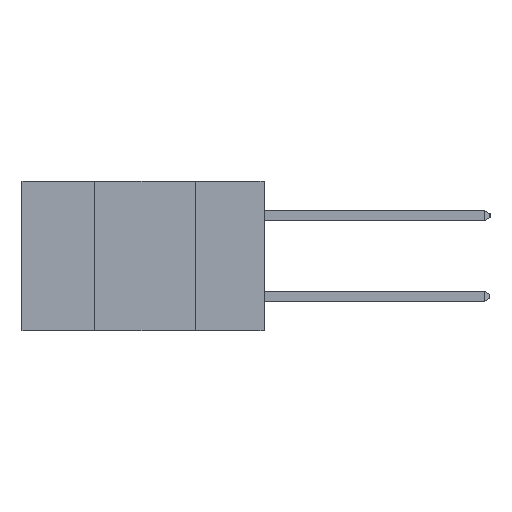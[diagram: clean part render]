
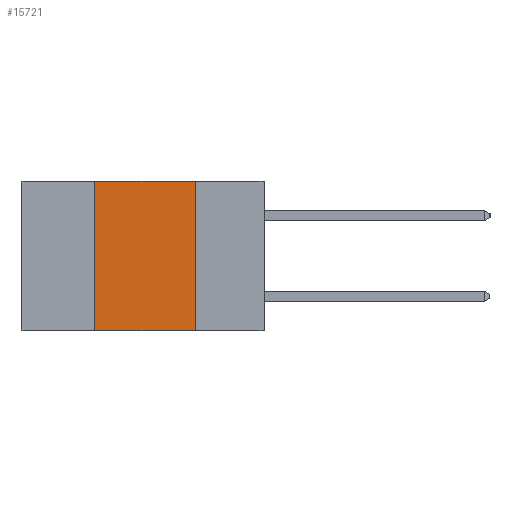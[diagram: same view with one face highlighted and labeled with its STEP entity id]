
A CAD part, left-side view. The second image highlights one B-rep face of the part: STEP entity #15721.
In plain terms, the highlighted planar face has unit normal (-1, 0, 0).
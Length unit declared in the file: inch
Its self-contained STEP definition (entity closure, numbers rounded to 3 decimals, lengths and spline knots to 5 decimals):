
#347 = VECTOR ( 'NONE', #2320, 39.37008 ) ;
#402 = DIRECTION ( 'NONE',  ( 0., 0., -1. ) ) ;
#819 = PLANE ( 'NONE',  #8789 ) ;
#997 = EDGE_CURVE ( 'NONE', #13735, #3631, #16819, .T. ) ;
#1044 = ORIENTED_EDGE ( 'NONE', *, *, #7484, .F. ) ;
#2320 = DIRECTION ( 'NONE',  ( 0., 0., -1. ) ) ;
#2417 = EDGE_LOOP ( 'NONE', ( #19217, #19425, #1044, #8109 ) ) ;
#3316 = CARTESIAN_POINT ( 'NONE',  ( 0., 0.42, -0.37 ) ) ;
#3631 = VERTEX_POINT ( 'NONE', #19331 ) ;
#3785 = CARTESIAN_POINT ( 'NONE',  ( 0., 0.6, -0.37 ) ) ;
#3962 = VECTOR ( 'NONE', #7563, 39.37008 ) ;
#4137 = EDGE_CURVE ( 'NONE', #11738, #3631, #20311, .T. ) ;
#5739 = DIRECTION ( 'NONE',  ( 0., 0., 1. ) ) ;
#7215 = CARTESIAN_POINT ( 'NONE',  ( 0., 0.17, -0.37 ) ) ;
#7484 = EDGE_CURVE ( 'NONE', #11738, #19159, #14266, .T. ) ;
#7563 = DIRECTION ( 'NONE',  ( 0., -1., 0. ) ) ;
#8109 = ORIENTED_EDGE ( 'NONE', *, *, #4137, .T. ) ;
#8789 = AXIS2_PLACEMENT_3D ( 'NONE', #18524, #15021, #402 ) ;
#9296 = VECTOR ( 'NONE', #5739, 39.37008 ) ;
#10312 = FACE_OUTER_BOUND ( 'NONE', #2417, .T. ) ;
#11537 = CARTESIAN_POINT ( 'NONE',  ( 0., 0.17, 0. ) ) ;
#11738 = VERTEX_POINT ( 'NONE', #3316 ) ;
#13527 = EDGE_CURVE ( 'NONE', #19159, #13735, #14410, .T. ) ;
#13735 = VERTEX_POINT ( 'NONE', #11537 ) ;
#13929 = DIRECTION ( 'NONE',  ( 0., -1., 0. ) ) ;
#14266 = LINE ( 'NONE', #20747, #9296 ) ;
#14410 = LINE ( 'NONE', #20885, #3962 ) ;
#14633 = CARTESIAN_POINT ( 'NONE',  ( 0., 0.42, 0. ) ) ;
#15021 = DIRECTION ( 'NONE',  ( 1., 0., 0. ) ) ;
#15721 = ADVANCED_FACE ( 'NONE', ( #10312 ), #819, .F. ) ;
#16819 = LINE ( 'NONE', #7215, #347 ) ;
#17655 = VECTOR ( 'NONE', #13929, 39.37008 ) ;
#18524 = CARTESIAN_POINT ( 'NONE',  ( 0., 0.6, 0. ) ) ;
#19159 = VERTEX_POINT ( 'NONE', #14633 ) ;
#19217 = ORIENTED_EDGE ( 'NONE', *, *, #997, .F. ) ;
#19331 = CARTESIAN_POINT ( 'NONE',  ( 0., 0.17, -0.37 ) ) ;
#19425 = ORIENTED_EDGE ( 'NONE', *, *, #13527, .F. ) ;
#20311 = LINE ( 'NONE', #3785, #17655 ) ;
#20747 = CARTESIAN_POINT ( 'NONE',  ( 0., 0.42, -0.37 ) ) ;
#20885 = CARTESIAN_POINT ( 'NONE',  ( 0., 0.6, 0. ) ) ;
